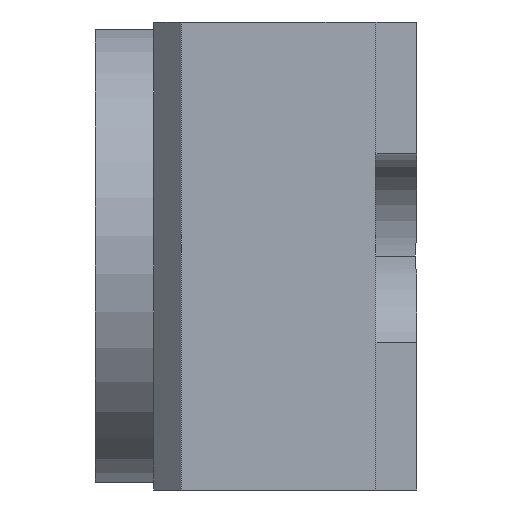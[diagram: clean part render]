
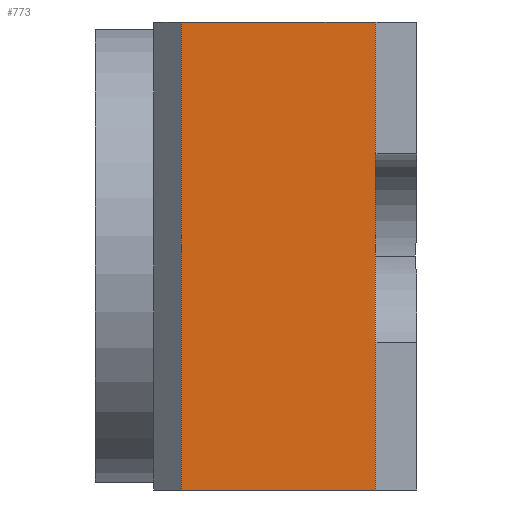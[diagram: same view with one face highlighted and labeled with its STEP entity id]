
A CAD part, front view. The second image highlights one B-rep face of the part: STEP entity #773.
In plain terms, the highlighted planar face has unit normal (0, -1, 0).
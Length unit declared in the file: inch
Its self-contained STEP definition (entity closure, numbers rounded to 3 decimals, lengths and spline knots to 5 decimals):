
#23 = VECTOR ( 'NONE', #731, 39.37008 ) ;
#33 = CARTESIAN_POINT ( 'NONE',  ( -0.79439, -0.257, 0.6 ) ) ;
#35 = EDGE_LOOP ( 'NONE', ( #171, #1012, #824, #53 ) ) ;
#36 = DIRECTION ( 'NONE',  ( 0., 0., 1. ) ) ;
#53 = ORIENTED_EDGE ( 'NONE', *, *, #190, .T. ) ;
#101 = CARTESIAN_POINT ( 'NONE',  ( -0.54575, -0.257, 0.6 ) ) ;
#105 = EDGE_CURVE ( 'NONE', #444, #225, #1050, .T. ) ;
#110 = DIRECTION ( 'NONE',  ( 0., 1., 0. ) ) ;
#146 = AXIS2_PLACEMENT_3D ( 'NONE', #291, #110, #36 ) ;
#171 = ORIENTED_EDGE ( 'NONE', *, *, #709, .T. ) ;
#184 = CARTESIAN_POINT ( 'NONE',  ( -0.79439, -0.257, 0.6 ) ) ;
#186 = VECTOR ( 'NONE', #512, 39.37008 ) ;
#190 = EDGE_CURVE ( 'NONE', #444, #283, #1013, .T. ) ;
#225 = VERTEX_POINT ( 'NONE', #101 ) ;
#283 = VERTEX_POINT ( 'NONE', #722 ) ;
#291 = CARTESIAN_POINT ( 'NONE',  ( -0.79439, -0.257, 0.6 ) ) ;
#298 = EDGE_CURVE ( 'NONE', #225, #468, #475, .T. ) ;
#316 = FACE_OUTER_BOUND ( 'NONE', #35, .T. ) ;
#440 = CARTESIAN_POINT ( 'NONE',  ( -0.79439, -0.257, 0. ) ) ;
#444 = VERTEX_POINT ( 'NONE', #744 ) ;
#468 = VERTEX_POINT ( 'NONE', #570 ) ;
#472 = CARTESIAN_POINT ( 'NONE',  ( -0.54575, -0.257, 0.6 ) ) ;
#475 = LINE ( 'NONE', #472, #23 ) ;
#512 = DIRECTION ( 'NONE',  ( 1., 0., 0. ) ) ;
#570 = CARTESIAN_POINT ( 'NONE',  ( -0.54575, -0.257, 0. ) ) ;
#614 = DIRECTION ( 'NONE',  ( 1., 0., 0. ) ) ;
#709 = EDGE_CURVE ( 'NONE', #283, #468, #1025, .T. ) ;
#711 = VECTOR ( 'NONE', #885, 39.37008 ) ;
#722 = CARTESIAN_POINT ( 'NONE',  ( -0.79439, -0.257, 0. ) ) ;
#731 = DIRECTION ( 'NONE',  ( 0., 0., -1. ) ) ;
#744 = CARTESIAN_POINT ( 'NONE',  ( -0.79439, -0.257, 0.6 ) ) ;
#773 = ADVANCED_FACE ( 'NONE', ( #316 ), #806, .F. ) ;
#806 = PLANE ( 'NONE',  #146 ) ;
#824 = ORIENTED_EDGE ( 'NONE', *, *, #105, .F. ) ;
#885 = DIRECTION ( 'NONE',  ( 0., 0., -1. ) ) ;
#955 = VECTOR ( 'NONE', #614, 39.37008 ) ;
#1012 = ORIENTED_EDGE ( 'NONE', *, *, #298, .F. ) ;
#1013 = LINE ( 'NONE', #33, #711 ) ;
#1025 = LINE ( 'NONE', #440, #955 ) ;
#1050 = LINE ( 'NONE', #184, #186 ) ;
